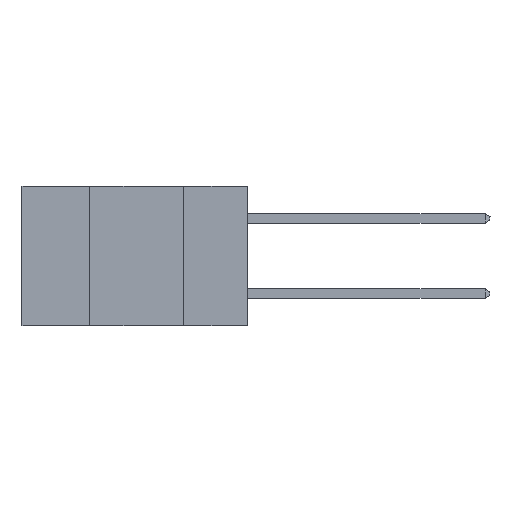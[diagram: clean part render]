
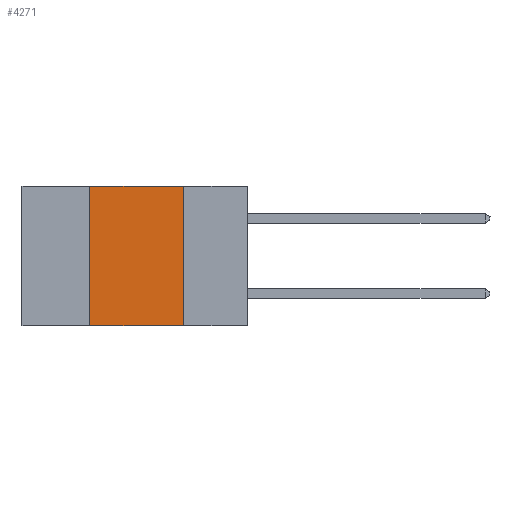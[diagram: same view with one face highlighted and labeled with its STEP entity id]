
A CAD part, left-side view. The second image highlights one B-rep face of the part: STEP entity #4271.
In plain terms, the highlighted planar face has unit normal (-1, 0, 0).
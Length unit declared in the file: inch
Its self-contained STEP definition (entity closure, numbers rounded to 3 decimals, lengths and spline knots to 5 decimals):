
#1206 = VERTEX_POINT ( 'NONE', #8542 ) ;
#1477 = FACE_OUTER_BOUND ( 'NONE', #19937, .T. ) ;
#2716 = AXIS2_PLACEMENT_3D ( 'NONE', #6317, #13232, #20005 ) ;
#3129 = LINE ( 'NONE', #3794, #12267 ) ;
#3701 = VERTEX_POINT ( 'NONE', #5866 ) ;
#3794 = CARTESIAN_POINT ( 'NONE',  ( 0., 0.17, 0. ) ) ;
#3946 = LINE ( 'NONE', #6751, #4239 ) ;
#4239 = VECTOR ( 'NONE', #10077, 39.37008 ) ;
#4271 = ADVANCED_FACE ( 'NONE', ( #1477 ), #7914, .F. ) ;
#5156 = LINE ( 'NONE', #5863, #17825 ) ;
#5863 = CARTESIAN_POINT ( 'NONE',  ( 0., 0.6, -0.37 ) ) ;
#5866 = CARTESIAN_POINT ( 'NONE',  ( 0., 0.17, 0. ) ) ;
#6264 = ORIENTED_EDGE ( 'NONE', *, *, #11510, .T. ) ;
#6317 = CARTESIAN_POINT ( 'NONE',  ( 0., 0.6, 0. ) ) ;
#6751 = CARTESIAN_POINT ( 'NONE',  ( 0., 0.6, 0. ) ) ;
#7001 = CARTESIAN_POINT ( 'NONE',  ( 0., 0.42, 0. ) ) ;
#7914 = PLANE ( 'NONE',  #2716 ) ;
#8173 = EDGE_CURVE ( 'NONE', #3701, #13938, #3129, .T. ) ;
#8542 = CARTESIAN_POINT ( 'NONE',  ( 0., 0.42, -0.37 ) ) ;
#9112 = VERTEX_POINT ( 'NONE', #16349 ) ;
#10077 = DIRECTION ( 'NONE',  ( 0., -1., 0. ) ) ;
#10797 = DIRECTION ( 'NONE',  ( 0., 0., -1. ) ) ;
#11510 = EDGE_CURVE ( 'NONE', #1206, #13938, #5156, .T. ) ;
#12122 = EDGE_CURVE ( 'NONE', #1206, #9112, #15562, .T. ) ;
#12267 = VECTOR ( 'NONE', #10797, 39.37008 ) ;
#12635 = EDGE_CURVE ( 'NONE', #9112, #3701, #3946, .T. ) ;
#13232 = DIRECTION ( 'NONE',  ( 1., 0., 0. ) ) ;
#13845 = DIRECTION ( 'NONE',  ( 0., 0., 1. ) ) ;
#13938 = VERTEX_POINT ( 'NONE', #19780 ) ;
#15562 = LINE ( 'NONE', #7001, #21498 ) ;
#16349 = CARTESIAN_POINT ( 'NONE',  ( 0., 0.42, 0. ) ) ;
#17238 = ORIENTED_EDGE ( 'NONE', *, *, #12122, .F. ) ;
#17825 = VECTOR ( 'NONE', #19681, 39.37008 ) ;
#19598 = ORIENTED_EDGE ( 'NONE', *, *, #8173, .F. ) ;
#19681 = DIRECTION ( 'NONE',  ( 0., -1., 0. ) ) ;
#19780 = CARTESIAN_POINT ( 'NONE',  ( 0., 0.17, -0.37 ) ) ;
#19937 = EDGE_LOOP ( 'NONE', ( #19598, #20748, #17238, #6264 ) ) ;
#20005 = DIRECTION ( 'NONE',  ( 0., 0., -1. ) ) ;
#20748 = ORIENTED_EDGE ( 'NONE', *, *, #12635, .F. ) ;
#21498 = VECTOR ( 'NONE', #13845, 39.37008 ) ;
